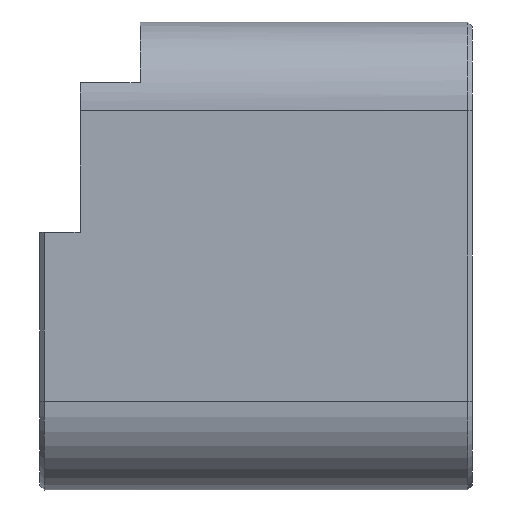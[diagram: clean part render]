
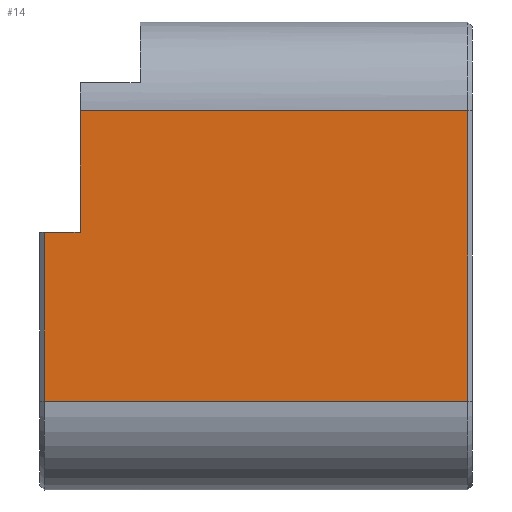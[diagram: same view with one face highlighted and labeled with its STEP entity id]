
A CAD part, left-side view. The second image highlights one B-rep face of the part: STEP entity #14.
In plain terms, the highlighted planar face has unit normal (-1, 0, 0).
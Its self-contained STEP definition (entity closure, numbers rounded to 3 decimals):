
#14 = ADVANCED_FACE ( 'NONE', ( #845 ), #800, .T. ) ;
#34 = ORIENTED_EDGE ( 'NONE', *, *, #808, .T. ) ;
#141 = CARTESIAN_POINT ( 'NONE',  ( -2.438, -0.127, -10.439 ) ) ;
#176 = VECTOR ( 'NONE', #487, 1000. ) ;
#210 = LINE ( 'NONE', #523, #176 ) ;
#223 = VERTEX_POINT ( 'NONE', #830 ) ;
#235 = CARTESIAN_POINT ( 'NONE',  ( -2.438, -11.913, -10.439 ) ) ;
#269 = CARTESIAN_POINT ( 'NONE',  ( -2.438, -1.118, -5.791 ) ) ;
#273 = VECTOR ( 'NONE', #807, 1000. ) ;
#274 = LINE ( 'NONE', #434, #273 ) ;
#277 = VECTOR ( 'NONE', #822, 1000. ) ;
#281 = LINE ( 'NONE', #835, #277 ) ;
#282 = VECTOR ( 'NONE', #886, 1000. ) ;
#284 = LINE ( 'NONE', #881, #282 ) ;
#300 = VECTOR ( 'NONE', #973, 1000. ) ;
#301 = LINE ( 'NONE', #269, #300 ) ;
#312 = VECTOR ( 'NONE', #402, 1000. ) ;
#313 = LINE ( 'NONE', #542, #312 ) ;
#402 = DIRECTION ( 'NONE',  ( 0., 0., 1. ) ) ;
#434 = CARTESIAN_POINT ( 'NONE',  ( -2.438, -11.913, -10.439 ) ) ;
#443 = VERTEX_POINT ( 'NONE', #707 ) ;
#487 = DIRECTION ( 'NONE',  ( 0., 1., 0. ) ) ;
#509 = ORIENTED_EDGE ( 'NONE', *, *, #853, .T. ) ;
#511 = ORIENTED_EDGE ( 'NONE', *, *, #861, .T. ) ;
#513 = ORIENTED_EDGE ( 'NONE', *, *, #914, .F. ) ;
#523 = CARTESIAN_POINT ( 'NONE',  ( -2.438, -11.913, -2.438 ) ) ;
#528 = ORIENTED_EDGE ( 'NONE', *, *, #637, .T. ) ;
#532 = ORIENTED_EDGE ( 'NONE', *, *, #969, .T. ) ;
#542 = CARTESIAN_POINT ( 'NONE',  ( -2.438, -11.786, -2.438 ) ) ;
#548 = VERTEX_POINT ( 'NONE', #716 ) ;
#605 = EDGE_LOOP ( 'NONE', ( #509, #511, #513, #528, #532, #34 ) ) ;
#637 = EDGE_CURVE ( 'NONE', #223, #443, #313, .T. ) ;
#640 = DIRECTION ( 'NONE',  ( 0., 0., 1. ) ) ;
#679 = DIRECTION ( 'NONE',  ( -1., 0., 0. ) ) ;
#707 = CARTESIAN_POINT ( 'NONE',  ( -2.438, -11.786, -2.438 ) ) ;
#716 = CARTESIAN_POINT ( 'NONE',  ( -2.438, -0.127, -5.791 ) ) ;
#747 = VERTEX_POINT ( 'NONE', #141 ) ;
#800 = PLANE ( 'NONE',  #901 ) ;
#807 = DIRECTION ( 'NONE',  ( 0., 1., 0. ) ) ;
#808 = EDGE_CURVE ( 'NONE', #827, #909, #301, .T. ) ;
#822 = DIRECTION ( 'NONE',  ( 0., 0., -1. ) ) ;
#827 = VERTEX_POINT ( 'NONE', #947 ) ;
#830 = CARTESIAN_POINT ( 'NONE',  ( -2.438, -11.786, -10.439 ) ) ;
#835 = CARTESIAN_POINT ( 'NONE',  ( -2.438, -0.127, -10.439 ) ) ;
#845 = FACE_OUTER_BOUND ( 'NONE', #605, .T. ) ;
#853 = EDGE_CURVE ( 'NONE', #909, #548, #284, .T. ) ;
#860 = CARTESIAN_POINT ( 'NONE',  ( -2.438, -1.118, -5.791 ) ) ;
#861 = EDGE_CURVE ( 'NONE', #548, #747, #281, .T. ) ;
#881 = CARTESIAN_POINT ( 'NONE',  ( -2.438, 0., -5.791 ) ) ;
#886 = DIRECTION ( 'NONE',  ( 0., 1., 0. ) ) ;
#901 = AXIS2_PLACEMENT_3D ( 'NONE', #235, #679, #640 ) ;
#909 = VERTEX_POINT ( 'NONE', #860 ) ;
#914 = EDGE_CURVE ( 'NONE', #223, #747, #274, .T. ) ;
#947 = CARTESIAN_POINT ( 'NONE',  ( -2.438, -1.118, -2.438 ) ) ;
#969 = EDGE_CURVE ( 'NONE', #443, #827, #210, .T. ) ;
#973 = DIRECTION ( 'NONE',  ( 0., 0., -1. ) ) ;
